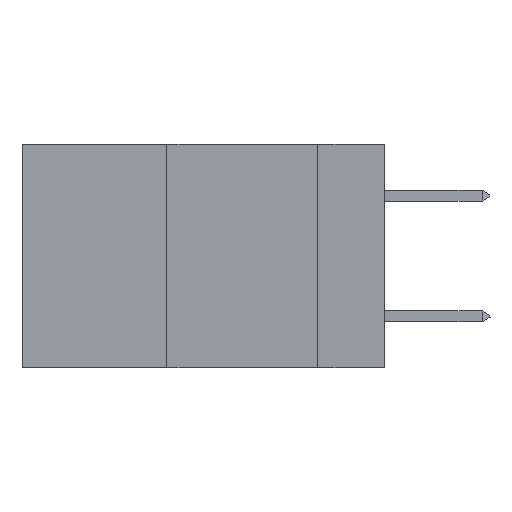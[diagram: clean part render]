
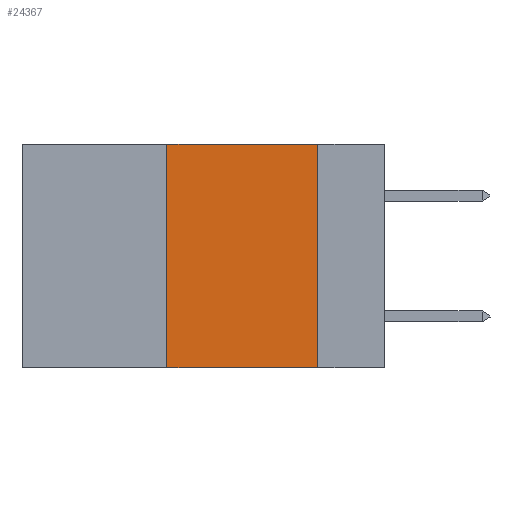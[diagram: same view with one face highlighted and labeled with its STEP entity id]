
A CAD part, left-side view. The second image highlights one B-rep face of the part: STEP entity #24367.
In plain terms, the highlighted planar face has unit normal (-1, 0, 0).
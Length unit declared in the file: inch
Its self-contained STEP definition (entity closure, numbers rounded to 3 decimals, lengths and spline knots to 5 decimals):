
#276 = VERTEX_POINT ( 'NONE', #4276 ) ;
#292 = VERTEX_POINT ( 'NONE', #25037 ) ;
#2539 = LINE ( 'NONE', #24021, #21536 ) ;
#3326 = ORIENTED_EDGE ( 'NONE', *, *, #19815, .F. ) ;
#3925 = VERTEX_POINT ( 'NONE', #15031 ) ;
#4276 = CARTESIAN_POINT ( 'NONE',  ( 0., 0.11, 0. ) ) ;
#5187 = CARTESIAN_POINT ( 'NONE',  ( 0., 0.6, -0.37 ) ) ;
#5266 = EDGE_CURVE ( 'NONE', #19995, #292, #24931, .T. ) ;
#5998 = EDGE_LOOP ( 'NONE', ( #19428, #3326, #21081, #6384 ) ) ;
#6384 = ORIENTED_EDGE ( 'NONE', *, *, #13190, .T. ) ;
#7154 = DIRECTION ( 'NONE',  ( 0., -1., 0. ) ) ;
#9889 = PLANE ( 'NONE',  #14277 ) ;
#10014 = CARTESIAN_POINT ( 'NONE',  ( 0., 0.36, -0.37 ) ) ;
#10531 = VECTOR ( 'NONE', #23716, 39.37008 ) ;
#11128 = VECTOR ( 'NONE', #7154, 39.37008 ) ;
#13190 = EDGE_CURVE ( 'NONE', #19995, #3925, #19766, .T. ) ;
#13952 = VECTOR ( 'NONE', #16797, 39.37008 ) ;
#14277 = AXIS2_PLACEMENT_3D ( 'NONE', #23840, #15883, #18014 ) ;
#15031 = CARTESIAN_POINT ( 'NONE',  ( 0., 0.11, -0.37 ) ) ;
#15883 = DIRECTION ( 'NONE',  ( 1., 0., 0. ) ) ;
#16132 = FACE_OUTER_BOUND ( 'NONE', #5998, .T. ) ;
#16797 = DIRECTION ( 'NONE',  ( 0., -1., 0. ) ) ;
#17076 = DIRECTION ( 'NONE',  ( 0., 0., -1. ) ) ;
#18014 = DIRECTION ( 'NONE',  ( 0., 0., -1. ) ) ;
#19428 = ORIENTED_EDGE ( 'NONE', *, *, #21144, .F. ) ;
#19766 = LINE ( 'NONE', #5187, #13952 ) ;
#19815 = EDGE_CURVE ( 'NONE', #292, #276, #21261, .T. ) ;
#19995 = VERTEX_POINT ( 'NONE', #10014 ) ;
#20706 = CARTESIAN_POINT ( 'NONE',  ( 0., 0.36, 0. ) ) ;
#21081 = ORIENTED_EDGE ( 'NONE', *, *, #5266, .F. ) ;
#21144 = EDGE_CURVE ( 'NONE', #276, #3925, #2539, .T. ) ;
#21261 = LINE ( 'NONE', #22661, #11128 ) ;
#21536 = VECTOR ( 'NONE', #17076, 39.37008 ) ;
#22661 = CARTESIAN_POINT ( 'NONE',  ( 0., 0.6, 0. ) ) ;
#23716 = DIRECTION ( 'NONE',  ( 0., 0., 1. ) ) ;
#23840 = CARTESIAN_POINT ( 'NONE',  ( 0., 0.6, 0. ) ) ;
#24021 = CARTESIAN_POINT ( 'NONE',  ( 0., 0.11, 0. ) ) ;
#24367 = ADVANCED_FACE ( 'NONE', ( #16132 ), #9889, .F. ) ;
#24931 = LINE ( 'NONE', #20706, #10531 ) ;
#25037 = CARTESIAN_POINT ( 'NONE',  ( 0., 0.36, 0. ) ) ;
